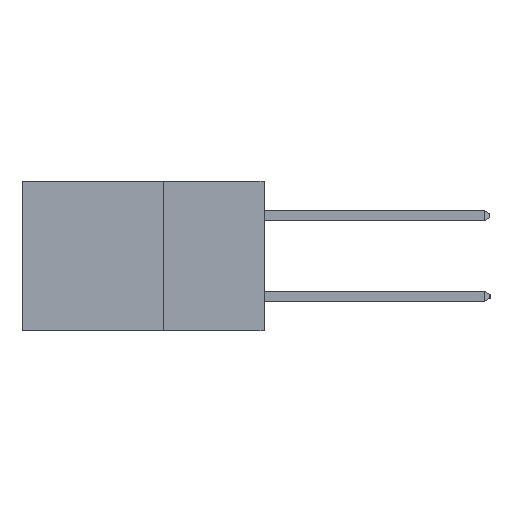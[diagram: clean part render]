
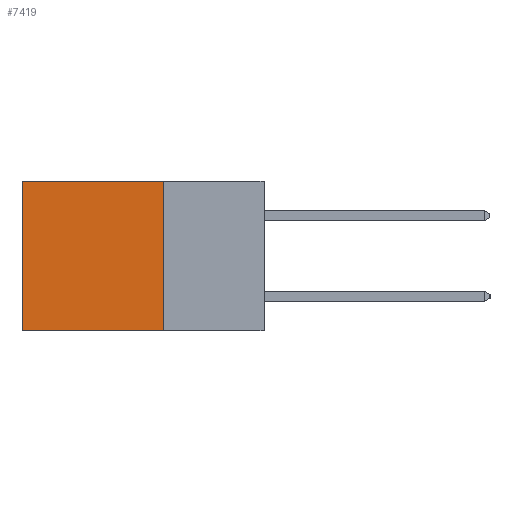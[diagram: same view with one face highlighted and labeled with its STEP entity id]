
A CAD part, left-side view. The second image highlights one B-rep face of the part: STEP entity #7419.
In plain terms, the highlighted planar face has unit normal (-1, 0, 0).
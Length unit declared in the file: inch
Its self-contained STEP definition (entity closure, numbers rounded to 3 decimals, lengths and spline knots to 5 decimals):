
#397 = CARTESIAN_POINT ( 'NONE',  ( 0.2615, 0.25, 0. ) ) ;
#1441 = VECTOR ( 'NONE', #11542, 39.37008 ) ;
#2299 = VECTOR ( 'NONE', #3881, 39.37008 ) ;
#2460 = EDGE_CURVE ( 'NONE', #11384, #14311, #13741, .T. ) ;
#2706 = VERTEX_POINT ( 'NONE', #5108 ) ;
#3100 = DIRECTION ( 'NONE',  ( 0., 1., 0. ) ) ;
#3645 = CARTESIAN_POINT ( 'NONE',  ( 0.2615, 0.25, 0. ) ) ;
#3881 = DIRECTION ( 'NONE',  ( 0., 1., 0. ) ) ;
#4025 = EDGE_CURVE ( 'NONE', #2706, #14138, #14632, .T. ) ;
#4118 = VECTOR ( 'NONE', #6576, 39.37008 ) ;
#4462 = LINE ( 'NONE', #6640, #4118 ) ;
#5108 = CARTESIAN_POINT ( 'NONE',  ( 0.2615, 0.25, -0.37 ) ) ;
#6058 = EDGE_LOOP ( 'NONE', ( #14529, #7064, #6234, #12524 ) ) ;
#6234 = ORIENTED_EDGE ( 'NONE', *, *, #9770, .F. ) ;
#6576 = DIRECTION ( 'NONE',  ( 0., 0., -1. ) ) ;
#6640 = CARTESIAN_POINT ( 'NONE',  ( 0.2615, 0.25, -0.37 ) ) ;
#7064 = ORIENTED_EDGE ( 'NONE', *, *, #4025, .F. ) ;
#7419 = ADVANCED_FACE ( 'NONE', ( #14210 ), #8054, .F. ) ;
#7460 = CARTESIAN_POINT ( 'NONE',  ( 0.2615, 0.25, -0.37 ) ) ;
#7967 = DIRECTION ( 'NONE',  ( 0., 0., -1. ) ) ;
#8034 = DIRECTION ( 'NONE',  ( 1., 0., 0. ) ) ;
#8054 = PLANE ( 'NONE',  #13574 ) ;
#8193 = CARTESIAN_POINT ( 'NONE',  ( 0.2615, 0.25, -0.37 ) ) ;
#9227 = VECTOR ( 'NONE', #3100, 39.37008 ) ;
#9770 = EDGE_CURVE ( 'NONE', #11384, #2706, #4462, .T. ) ;
#11384 = VERTEX_POINT ( 'NONE', #3645 ) ;
#11489 = CARTESIAN_POINT ( 'NONE',  ( 0.2615, 0.6, -0.37 ) ) ;
#11542 = DIRECTION ( 'NONE',  ( 0., 0., -1. ) ) ;
#12524 = ORIENTED_EDGE ( 'NONE', *, *, #2460, .T. ) ;
#12804 = CARTESIAN_POINT ( 'NONE',  ( 0.2615, 0.6, 0. ) ) ;
#13574 = AXIS2_PLACEMENT_3D ( 'NONE', #8193, #8034, #7967 ) ;
#13658 = LINE ( 'NONE', #11489, #1441 ) ;
#13741 = LINE ( 'NONE', #397, #2299 ) ;
#14138 = VERTEX_POINT ( 'NONE', #14356 ) ;
#14210 = FACE_OUTER_BOUND ( 'NONE', #6058, .T. ) ;
#14311 = VERTEX_POINT ( 'NONE', #12804 ) ;
#14356 = CARTESIAN_POINT ( 'NONE',  ( 0.2615, 0.6, -0.37 ) ) ;
#14467 = EDGE_CURVE ( 'NONE', #14311, #14138, #13658, .T. ) ;
#14529 = ORIENTED_EDGE ( 'NONE', *, *, #14467, .T. ) ;
#14632 = LINE ( 'NONE', #7460, #9227 ) ;
